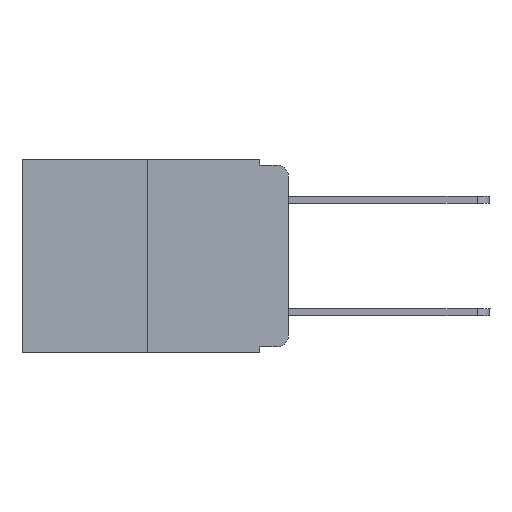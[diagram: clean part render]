
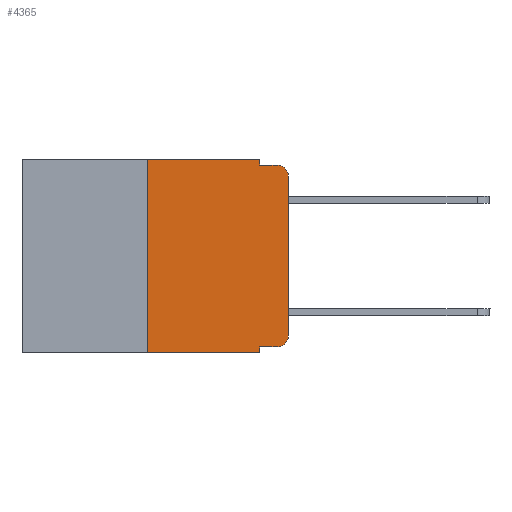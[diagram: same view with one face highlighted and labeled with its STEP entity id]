
A CAD part, left-side view. The second image highlights one B-rep face of the part: STEP entity #4365.
In plain terms, the highlighted planar face has unit normal (-1, 0, 0).
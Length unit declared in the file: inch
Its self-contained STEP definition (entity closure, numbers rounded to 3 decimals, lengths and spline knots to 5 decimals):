
#48 = CIRCLE ( 'NONE', #277, 0.02 ) ;
#219 = CIRCLE ( 'NONE', #9966, 0.02 ) ;
#231 = VERTEX_POINT ( 'NONE', #6327 ) ;
#277 = AXIS2_PLACEMENT_3D ( 'NONE', #1169, #12840, #3148 ) ;
#364 = AXIS2_PLACEMENT_3D ( 'NONE', #11816, #10763, #6645 ) ;
#831 = VERTEX_POINT ( 'NONE', #11563 ) ;
#875 = EDGE_LOOP ( 'NONE', ( #5200, #9750, #9557, #12041, #1955, #1758, #4866, #3519, #11406, #7086 ) ) ;
#1038 = EDGE_CURVE ( 'NONE', #7024, #1477, #1755, .T. ) ;
#1169 = CARTESIAN_POINT ( 'NONE',  ( 0., 0.02, -0.313 ) ) ;
#1289 = LINE ( 'NONE', #8787, #9924 ) ;
#1333 = LINE ( 'NONE', #5720, #12651 ) ;
#1406 = CARTESIAN_POINT ( 'NONE',  ( 0., 0., -0.03 ) ) ;
#1440 = DIRECTION ( 'NONE',  ( 0., 0., -1. ) ) ;
#1477 = VERTEX_POINT ( 'NONE', #5907 ) ;
#1755 = LINE ( 'NONE', #11236, #2992 ) ;
#1758 = ORIENTED_EDGE ( 'NONE', *, *, #1038, .F. ) ;
#1955 = ORIENTED_EDGE ( 'NONE', *, *, #13915, .F. ) ;
#2145 = LINE ( 'NONE', #11707, #6550 ) ;
#2552 = VECTOR ( 'NONE', #1440, 39.37008 ) ;
#2761 = LINE ( 'NONE', #13733, #6511 ) ;
#2992 = VECTOR ( 'NONE', #12513, 39.37008 ) ;
#3139 = EDGE_CURVE ( 'NONE', #831, #3244, #13559, .T. ) ;
#3148 = DIRECTION ( 'NONE',  ( 0., 0., -1. ) ) ;
#3221 = CARTESIAN_POINT ( 'NONE',  ( 0., 0., -0.313 ) ) ;
#3244 = VERTEX_POINT ( 'NONE', #13416 ) ;
#3519 = ORIENTED_EDGE ( 'NONE', *, *, #11341, .F. ) ;
#4020 = LINE ( 'NONE', #8349, #8384 ) ;
#4365 = ADVANCED_FACE ( 'NONE', ( #8556 ), #7502, .F. ) ;
#4440 = DIRECTION ( 'NONE',  ( 0., 0., -1. ) ) ;
#4641 = CARTESIAN_POINT ( 'NONE',  ( 0., 0.25, -0.343 ) ) ;
#4866 = ORIENTED_EDGE ( 'NONE', *, *, #11843, .T. ) ;
#5200 = ORIENTED_EDGE ( 'NONE', *, *, #12965, .T. ) ;
#5458 = LINE ( 'NONE', #10855, #13583 ) ;
#5508 = DIRECTION ( 'NONE',  ( -1., 0., 0. ) ) ;
#5720 = CARTESIAN_POINT ( 'NONE',  ( 0., 0.051, -0.333 ) ) ;
#5907 = CARTESIAN_POINT ( 'NONE',  ( 0., 0.25, 0. ) ) ;
#6327 = CARTESIAN_POINT ( 'NONE',  ( 0., 0.02, -0.333 ) ) ;
#6511 = VECTOR ( 'NONE', #11537, 39.37008 ) ;
#6528 = VERTEX_POINT ( 'NONE', #3221 ) ;
#6550 = VECTOR ( 'NONE', #13914, 39.37008 ) ;
#6645 = DIRECTION ( 'NONE',  ( 0., 0., -1. ) ) ;
#6796 = CARTESIAN_POINT ( 'NONE',  ( 0., 0.02, -0.03 ) ) ;
#6956 = EDGE_CURVE ( 'NONE', #8716, #231, #1333, .T. ) ;
#7024 = VERTEX_POINT ( 'NONE', #4641 ) ;
#7086 = ORIENTED_EDGE ( 'NONE', *, *, #7513, .T. ) ;
#7502 = PLANE ( 'NONE',  #364 ) ;
#7513 = EDGE_CURVE ( 'NONE', #231, #6528, #48, .T. ) ;
#7534 = DIRECTION ( 'NONE',  ( 0., -1., 0. ) ) ;
#8349 = CARTESIAN_POINT ( 'NONE',  ( 0., 0.473, 0. ) ) ;
#8384 = VECTOR ( 'NONE', #10688, 39.37008 ) ;
#8556 = FACE_OUTER_BOUND ( 'NONE', #875, .T. ) ;
#8716 = VERTEX_POINT ( 'NONE', #10468 ) ;
#8769 = CARTESIAN_POINT ( 'NONE',  ( 0., 0.051, -0.343 ) ) ;
#8787 = CARTESIAN_POINT ( 'NONE',  ( 0., 0.473, -0.343 ) ) ;
#9557 = ORIENTED_EDGE ( 'NONE', *, *, #13043, .F. ) ;
#9750 = ORIENTED_EDGE ( 'NONE', *, *, #13680, .T. ) ;
#9924 = VECTOR ( 'NONE', #10984, 39.37008 ) ;
#9966 = AXIS2_PLACEMENT_3D ( 'NONE', #6796, #5508, #4440 ) ;
#10468 = CARTESIAN_POINT ( 'NONE',  ( 0., 0.051, -0.333 ) ) ;
#10688 = DIRECTION ( 'NONE',  ( 0., -1., 0. ) ) ;
#10763 = DIRECTION ( 'NONE',  ( 1., 0., 0. ) ) ;
#10787 = CARTESIAN_POINT ( 'NONE',  ( 0., 0.02, -0.01 ) ) ;
#10855 = CARTESIAN_POINT ( 'NONE',  ( 0., 0.051, -0.01 ) ) ;
#10984 = DIRECTION ( 'NONE',  ( 0., -1., 0. ) ) ;
#11176 = VERTEX_POINT ( 'NONE', #1406 ) ;
#11236 = CARTESIAN_POINT ( 'NONE',  ( 0., 0.25, 0. ) ) ;
#11341 = EDGE_CURVE ( 'NONE', #8716, #13719, #2761, .T. ) ;
#11363 = CARTESIAN_POINT ( 'NONE',  ( 0., 0.051, 0. ) ) ;
#11406 = ORIENTED_EDGE ( 'NONE', *, *, #6956, .T. ) ;
#11537 = DIRECTION ( 'NONE',  ( 0., 0., -1. ) ) ;
#11563 = CARTESIAN_POINT ( 'NONE',  ( 0., 0.051, 0. ) ) ;
#11707 = CARTESIAN_POINT ( 'NONE',  ( 0., 0., 0. ) ) ;
#11816 = CARTESIAN_POINT ( 'NONE',  ( 0., 0.473, 0. ) ) ;
#11817 = VERTEX_POINT ( 'NONE', #10787 ) ;
#11843 = EDGE_CURVE ( 'NONE', #7024, #13719, #1289, .T. ) ;
#12041 = ORIENTED_EDGE ( 'NONE', *, *, #3139, .F. ) ;
#12230 = DIRECTION ( 'NONE',  ( 0., -1., 0. ) ) ;
#12513 = DIRECTION ( 'NONE',  ( 0., 0., 1. ) ) ;
#12651 = VECTOR ( 'NONE', #12230, 39.37008 ) ;
#12840 = DIRECTION ( 'NONE',  ( -1., 0., 0. ) ) ;
#12965 = EDGE_CURVE ( 'NONE', #6528, #11176, #2145, .T. ) ;
#13043 = EDGE_CURVE ( 'NONE', #3244, #11817, #5458, .T. ) ;
#13416 = CARTESIAN_POINT ( 'NONE',  ( 0., 0.051, -0.01 ) ) ;
#13559 = LINE ( 'NONE', #11363, #2552 ) ;
#13583 = VECTOR ( 'NONE', #7534, 39.37008 ) ;
#13680 = EDGE_CURVE ( 'NONE', #11176, #11817, #219, .T. ) ;
#13719 = VERTEX_POINT ( 'NONE', #8769 ) ;
#13733 = CARTESIAN_POINT ( 'NONE',  ( 0., 0.051, 0. ) ) ;
#13914 = DIRECTION ( 'NONE',  ( 0., 0., 1. ) ) ;
#13915 = EDGE_CURVE ( 'NONE', #1477, #831, #4020, .T. ) ;
